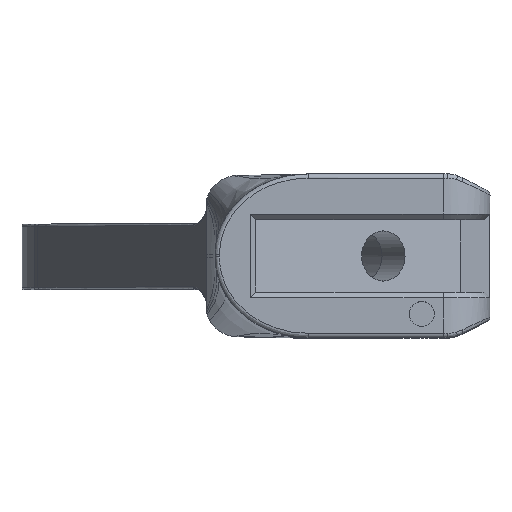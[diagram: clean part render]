
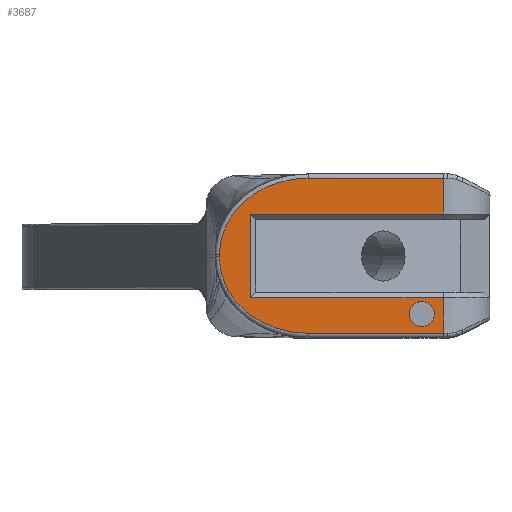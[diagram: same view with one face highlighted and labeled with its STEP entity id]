
A CAD part, top view. The second image highlights one B-rep face of the part: STEP entity #3687.
In plain terms, the highlighted planar face has unit normal (0, 0, 1).
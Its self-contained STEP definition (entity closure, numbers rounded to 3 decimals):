
#37=FACE_BOUND('',#989,.T.);
#176=B_SPLINE_CURVE_WITH_KNOTS('',3,(#8010,#8011,#8012,#8013,#8014,#8015,
#8016,#8017,#8018,#8019),.UNSPECIFIED.,.F.,.F.,(4,2,2,2,4),(0.,0.571,
0.976,1.452,1.75),.UNSPECIFIED.);
#177=B_SPLINE_CURVE_WITH_KNOTS('',3,(#8022,#8023,#8024,#8025,#8026,#8027,
#8028,#8029,#8030,#8031,#8032,#8033,#8034,#8035),.UNSPECIFIED.,.F.,.F.,
(4,2,2,2,2,2,4),(0.,0.148,0.479,0.833,
1.137,1.486,1.752),.UNSPECIFIED.);
#530=CIRCLE('',#4040,1.7);
#737=FACE_OUTER_BOUND('',#988,.T.);
#988=EDGE_LOOP('',(#2981,#2982,#2983,#2984,#2985,#2986,#2987,#2988,#2989,
#2990));
#989=EDGE_LOOP('',(#2991));
#1198=LINE('',#7871,#1372);
#1203=LINE('',#7999,#1377);
#1204=LINE('',#8001,#1378);
#1205=LINE('',#8003,#1379);
#1206=LINE('',#8005,#1380);
#1207=LINE('',#8006,#1381);
#1208=LINE('',#8008,#1382);
#1209=LINE('',#8021,#1383);
#1372=VECTOR('',#4714,10.);
#1377=VECTOR('',#4735,10.);
#1378=VECTOR('',#4736,10.);
#1379=VECTOR('',#4737,10.);
#1380=VECTOR('',#4738,10.);
#1381=VECTOR('',#4739,10.);
#1382=VECTOR('',#4740,10.);
#1383=VECTOR('',#4741,10.);
#1651=VERTEX_POINT('',#7867);
#1653=VERTEX_POINT('',#7870);
#1669=VERTEX_POINT('',#7997);
#1670=VERTEX_POINT('',#7998);
#1671=VERTEX_POINT('',#8000);
#1672=VERTEX_POINT('',#8002);
#1673=VERTEX_POINT('',#8004);
#1674=VERTEX_POINT('',#8007);
#1675=VERTEX_POINT('',#8009);
#1676=VERTEX_POINT('',#8020);
#1677=VERTEX_POINT('',#8036);
#2112=EDGE_CURVE('',#1651,#1653,#1198,.T.);
#2130=EDGE_CURVE('',#1669,#1670,#1203,.T.);
#2131=EDGE_CURVE('',#1669,#1671,#1204,.T.);
#2132=EDGE_CURVE('',#1672,#1671,#1205,.T.);
#2133=EDGE_CURVE('',#1673,#1672,#1206,.T.);
#2134=EDGE_CURVE('',#1653,#1673,#1207,.T.);
#2135=EDGE_CURVE('',#1674,#1651,#1208,.T.);
#2136=EDGE_CURVE('',#1675,#1674,#176,.T.);
#2137=EDGE_CURVE('',#1676,#1675,#1209,.T.);
#2138=EDGE_CURVE('',#1670,#1676,#177,.T.);
#2139=EDGE_CURVE('',#1677,#1677,#530,.T.);
#2981=ORIENTED_EDGE('',*,*,#2130,.F.);
#2982=ORIENTED_EDGE('',*,*,#2131,.T.);
#2983=ORIENTED_EDGE('',*,*,#2132,.F.);
#2984=ORIENTED_EDGE('',*,*,#2133,.F.);
#2985=ORIENTED_EDGE('',*,*,#2134,.F.);
#2986=ORIENTED_EDGE('',*,*,#2112,.F.);
#2987=ORIENTED_EDGE('',*,*,#2135,.F.);
#2988=ORIENTED_EDGE('',*,*,#2136,.F.);
#2989=ORIENTED_EDGE('',*,*,#2137,.F.);
#2990=ORIENTED_EDGE('',*,*,#2138,.F.);
#2991=ORIENTED_EDGE('',*,*,#2139,.T.);
#3539=PLANE('',#4039);
#3687=ADVANCED_FACE('',(#737,#37),#3539,.T.);
#4039=AXIS2_PLACEMENT_3D('',#7996,#4733,#4734);
#4040=AXIS2_PLACEMENT_3D('',#8037,#4742,#4743);
#4714=DIRECTION('',(0.,-1.,0.));
#4733=DIRECTION('center_axis',(0.,0.,
1.));
#4734=DIRECTION('ref_axis',(1.,0.,0.));
#4735=DIRECTION('',(-1.,0.,0.));
#4736=DIRECTION('',(0.,1.,0.));
#4737=DIRECTION('',(1.,0.,0.));
#4738=DIRECTION('',(0.,-1.,0.));
#4739=DIRECTION('',(-1.,0.,0.));
#4740=DIRECTION('',(1.,0.,0.));
#4741=DIRECTION('',(0.,1.,0.));
#4742=DIRECTION('center_axis',(0.,0.,
-1.));
#4743=DIRECTION('ref_axis',(0.,1.,0.));
#7867=CARTESIAN_POINT('',(-3.41,-21.904,42.306));
#7870=CARTESIAN_POINT('',(-3.41,-26.753,42.306));
#7871=CARTESIAN_POINT('',(-3.41,-37.292,42.306));
#7996=CARTESIAN_POINT('Origin',(-34.254,-37.291,42.305));
#7997=CARTESIAN_POINT('',(-3.41,-42.931,42.306));
#7998=CARTESIAN_POINT('',(-21.731,-42.931,42.306));
#7999=CARTESIAN_POINT('',(-27.992,-42.93,42.305));
#8000=CARTESIAN_POINT('',(-3.41,-38.082,42.306));
#8001=CARTESIAN_POINT('',(-3.41,-27.543,42.306));
#8002=CARTESIAN_POINT('',(-29.56,-38.081,42.305));
#8003=CARTESIAN_POINT('',(-32.259,-38.081,42.305));
#8004=CARTESIAN_POINT('',(-29.56,-26.753,42.305));
#8005=CARTESIAN_POINT('',(-29.56,-32.326,42.305));
#8006=CARTESIAN_POINT('',(-32.259,-26.753,42.305));
#8007=CARTESIAN_POINT('',(-21.73,-21.904,42.306));
#8008=CARTESIAN_POINT('',(-21.522,-21.904,42.306));
#8009=CARTESIAN_POINT('',(-33.751,-32.254,42.305));
#8010=CARTESIAN_POINT('Ctrl Pts',(-33.751,-32.254,42.305));
#8011=CARTESIAN_POINT('Ctrl Pts',(-33.751,-30.35,42.305));
#8012=CARTESIAN_POINT('Ctrl Pts',(-33.115,-28.459,42.305));
#8013=CARTESIAN_POINT('Ctrl Pts',(-31.224,-25.776,42.305));
#8014=CARTESIAN_POINT('Ctrl Pts',(-30.229,-24.833,42.305));
#8015=CARTESIAN_POINT('Ctrl Pts',(-27.763,-23.186,42.305));
#8016=CARTESIAN_POINT('Ctrl Pts',(-26.27,-22.57,42.305));
#8017=CARTESIAN_POINT('Ctrl Pts',(-23.726,-22.011,42.306));
#8018=CARTESIAN_POINT('Ctrl Pts',(-22.722,-21.904,42.306));
#8019=CARTESIAN_POINT('Ctrl Pts',(-21.73,-21.904,42.306));
#8020=CARTESIAN_POINT('',(-33.751,-32.58,42.305));
#8021=CARTESIAN_POINT('',(-33.751,-34.773,42.305));
#8022=CARTESIAN_POINT('Ctrl Pts',(-21.731,-42.931,42.306));
#8023=CARTESIAN_POINT('Ctrl Pts',(-22.224,-42.93,42.306));
#8024=CARTESIAN_POINT('Ctrl Pts',(-22.719,-42.904,42.306));
#8025=CARTESIAN_POINT('Ctrl Pts',(-24.31,-42.734,42.306));
#8026=CARTESIAN_POINT('Ctrl Pts',(-25.392,-42.486,42.305));
#8027=CARTESIAN_POINT('Ctrl Pts',(-27.545,-41.698,42.305));
#8028=CARTESIAN_POINT('Ctrl Pts',(-28.603,-41.14,42.305));
#8029=CARTESIAN_POINT('Ctrl Pts',(-30.381,-39.825,42.305));
#8030=CARTESIAN_POINT('Ctrl Pts',(-31.115,-39.117,42.305));
#8031=CARTESIAN_POINT('Ctrl Pts',(-32.454,-37.386,42.305));
#8032=CARTESIAN_POINT('Ctrl Pts',(-33.011,-36.336,42.305));
#8033=CARTESIAN_POINT('Ctrl Pts',(-33.615,-34.364,42.305));
#8034=CARTESIAN_POINT('Ctrl Pts',(-33.751,-33.466,42.305));
#8035=CARTESIAN_POINT('Ctrl Pts',(-33.751,-32.58,42.305));
#8036=CARTESIAN_POINT('',(-6.305,-41.994,42.306));
#8037=CARTESIAN_POINT('Origin',(-6.305,-40.294,42.306));
